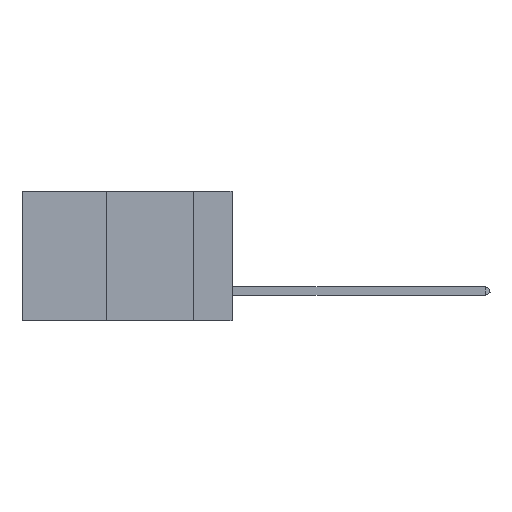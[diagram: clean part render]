
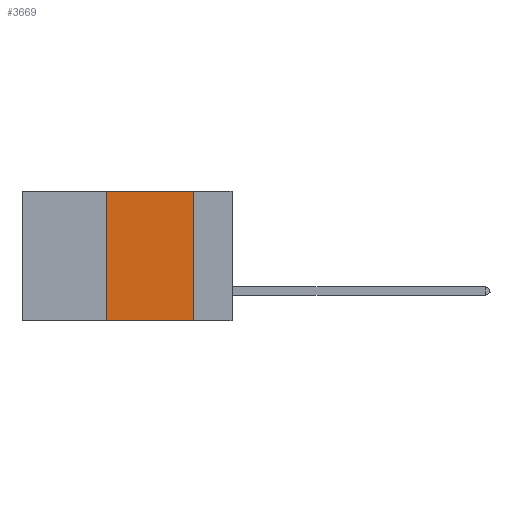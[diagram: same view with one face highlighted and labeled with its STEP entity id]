
A CAD part, left-side view. The second image highlights one B-rep face of the part: STEP entity #3669.
In plain terms, the highlighted planar face has unit normal (-1, 0, 0).
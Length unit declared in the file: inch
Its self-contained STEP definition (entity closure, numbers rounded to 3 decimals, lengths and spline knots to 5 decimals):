
#186 = CARTESIAN_POINT ( 'NONE',  ( 0., 0.36, 0. ) ) ;
#749 = CARTESIAN_POINT ( 'NONE',  ( 0., 0.6, -0.37 ) ) ;
#761 = ORIENTED_EDGE ( 'NONE', *, *, #18617, .F. ) ;
#1429 = DIRECTION ( 'NONE',  ( 0., 0., -1. ) ) ;
#1951 = VERTEX_POINT ( 'NONE', #18009 ) ;
#2210 = VERTEX_POINT ( 'NONE', #33043 ) ;
#3122 = EDGE_CURVE ( 'NONE', #2210, #42449, #30030, .T. ) ;
#3458 = VECTOR ( 'NONE', #1429, 39.37008 ) ;
#3669 = ADVANCED_FACE ( 'NONE', ( #37664 ), #29336, .F. ) ;
#10319 = VECTOR ( 'NONE', #18053, 39.37008 ) ;
#10871 = ORIENTED_EDGE ( 'NONE', *, *, #20330, .F. ) ;
#11213 = CARTESIAN_POINT ( 'NONE',  ( 0., 0.11, 0. ) ) ;
#12385 = VECTOR ( 'NONE', #27774, 39.37008 ) ;
#12788 = LINE ( 'NONE', #11213, #3458 ) ;
#15111 = ORIENTED_EDGE ( 'NONE', *, *, #3122, .T. ) ;
#17484 = DIRECTION ( 'NONE',  ( 0., 0., 1. ) ) ;
#18009 = CARTESIAN_POINT ( 'NONE',  ( 0., 0.36, 0. ) ) ;
#18053 = DIRECTION ( 'NONE',  ( 0., -1., 0. ) ) ;
#18617 = EDGE_CURVE ( 'NONE', #1951, #40392, #26627, .T. ) ;
#19973 = ORIENTED_EDGE ( 'NONE', *, *, #22094, .F. ) ;
#20330 = EDGE_CURVE ( 'NONE', #40392, #42449, #12788, .T. ) ;
#22094 = EDGE_CURVE ( 'NONE', #2210, #1951, #35954, .T. ) ;
#26627 = LINE ( 'NONE', #27177, #12385 ) ;
#27177 = CARTESIAN_POINT ( 'NONE',  ( 0., 0.6, 0. ) ) ;
#27774 = DIRECTION ( 'NONE',  ( 0., -1., 0. ) ) ;
#29336 = PLANE ( 'NONE',  #29612 ) ;
#29612 = AXIS2_PLACEMENT_3D ( 'NONE', #32429, #35928, #39459 ) ;
#30030 = LINE ( 'NONE', #749, #10319 ) ;
#32429 = CARTESIAN_POINT ( 'NONE',  ( 0., 0.6, 0. ) ) ;
#33043 = CARTESIAN_POINT ( 'NONE',  ( 0., 0.36, -0.37 ) ) ;
#35928 = DIRECTION ( 'NONE',  ( 1., 0., 0. ) ) ;
#35954 = LINE ( 'NONE', #186, #37065 ) ;
#37065 = VECTOR ( 'NONE', #17484, 39.37008 ) ;
#37664 = FACE_OUTER_BOUND ( 'NONE', #43889, .T. ) ;
#39459 = DIRECTION ( 'NONE',  ( 0., 0., -1. ) ) ;
#40323 = CARTESIAN_POINT ( 'NONE',  ( 0., 0.11, 0. ) ) ;
#40392 = VERTEX_POINT ( 'NONE', #40323 ) ;
#42449 = VERTEX_POINT ( 'NONE', #43137 ) ;
#43137 = CARTESIAN_POINT ( 'NONE',  ( 0., 0.11, -0.37 ) ) ;
#43889 = EDGE_LOOP ( 'NONE', ( #10871, #761, #19973, #15111 ) ) ;
